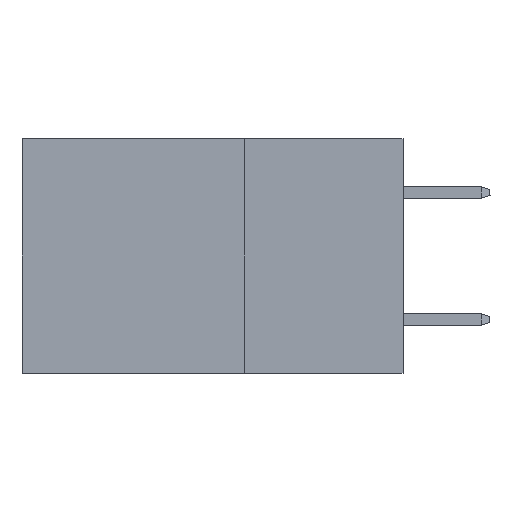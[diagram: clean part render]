
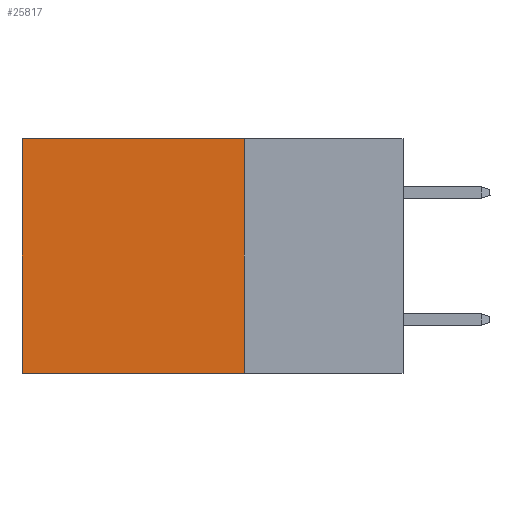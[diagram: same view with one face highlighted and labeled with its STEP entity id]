
A CAD part, left-side view. The second image highlights one B-rep face of the part: STEP entity #25817.
In plain terms, the highlighted planar face has unit normal (-1, 0, 0).
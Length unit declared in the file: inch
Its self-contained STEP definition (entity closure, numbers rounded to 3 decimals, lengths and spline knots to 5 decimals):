
#3070 = DIRECTION ( 'NONE',  ( 0., 0., -1. ) ) ;
#3986 = LINE ( 'NONE', #32331, #29122 ) ;
#5298 = DIRECTION ( 'NONE',  ( 0., 0., -1. ) ) ;
#6178 = CARTESIAN_POINT ( 'NONE',  ( 0.2875, 0.25, -0.37 ) ) ;
#7010 = EDGE_CURVE ( 'NONE', #29570, #13120, #3986, .T. ) ;
#7138 = DIRECTION ( 'NONE',  ( 0., 1., 0. ) ) ;
#7150 = LINE ( 'NONE', #35680, #35495 ) ;
#8986 = CARTESIAN_POINT ( 'NONE',  ( 0.2875, 0.6, -0.37 ) ) ;
#9329 = CARTESIAN_POINT ( 'NONE',  ( 0.2875, 0.6, 0. ) ) ;
#12623 = EDGE_LOOP ( 'NONE', ( #26934, #13072, #15592, #13115 ) ) ;
#12886 = EDGE_CURVE ( 'NONE', #22583, #21917, #7150, .T. ) ;
#13072 = ORIENTED_EDGE ( 'NONE', *, *, #7010, .F. ) ;
#13115 = ORIENTED_EDGE ( 'NONE', *, *, #12886, .T. ) ;
#13120 = VERTEX_POINT ( 'NONE', #8986 ) ;
#13496 = LINE ( 'NONE', #19461, #21333 ) ;
#14402 = DIRECTION ( 'NONE',  ( 1., 0., 0. ) ) ;
#14574 = CARTESIAN_POINT ( 'NONE',  ( 0.2875, 0.25, 0. ) ) ;
#14791 = LINE ( 'NONE', #34376, #24909 ) ;
#15592 = ORIENTED_EDGE ( 'NONE', *, *, #29094, .F. ) ;
#18518 = DIRECTION ( 'NONE',  ( 0., 1., 0. ) ) ;
#19461 = CARTESIAN_POINT ( 'NONE',  ( 0.2875, 0.25, 0. ) ) ;
#21333 = VECTOR ( 'NONE', #5298, 39.37008 ) ;
#21917 = VERTEX_POINT ( 'NONE', #9329 ) ;
#22583 = VERTEX_POINT ( 'NONE', #33870 ) ;
#24909 = VECTOR ( 'NONE', #3070, 39.37008 ) ;
#25404 = FACE_OUTER_BOUND ( 'NONE', #12623, .T. ) ;
#25817 = ADVANCED_FACE ( 'NONE', ( #25404 ), #31358, .F. ) ;
#26934 = ORIENTED_EDGE ( 'NONE', *, *, #29185, .T. ) ;
#29094 = EDGE_CURVE ( 'NONE', #22583, #29570, #13496, .T. ) ;
#29122 = VECTOR ( 'NONE', #7138, 39.37008 ) ;
#29185 = EDGE_CURVE ( 'NONE', #21917, #13120, #14791, .T. ) ;
#29570 = VERTEX_POINT ( 'NONE', #6178 ) ;
#31358 = PLANE ( 'NONE',  #33156 ) ;
#32331 = CARTESIAN_POINT ( 'NONE',  ( 0.2875, 0.25, -0.37 ) ) ;
#33156 = AXIS2_PLACEMENT_3D ( 'NONE', #14574, #14402, #33990 ) ;
#33870 = CARTESIAN_POINT ( 'NONE',  ( 0.2875, 0.25, 0. ) ) ;
#33990 = DIRECTION ( 'NONE',  ( 0., 0., -1. ) ) ;
#34376 = CARTESIAN_POINT ( 'NONE',  ( 0.2875, 0.6, 0. ) ) ;
#35495 = VECTOR ( 'NONE', #18518, 39.37008 ) ;
#35680 = CARTESIAN_POINT ( 'NONE',  ( 0.2875, 0.25, 0. ) ) ;
